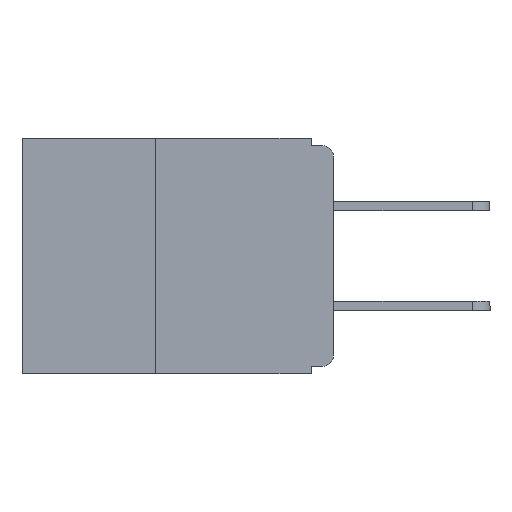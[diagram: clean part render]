
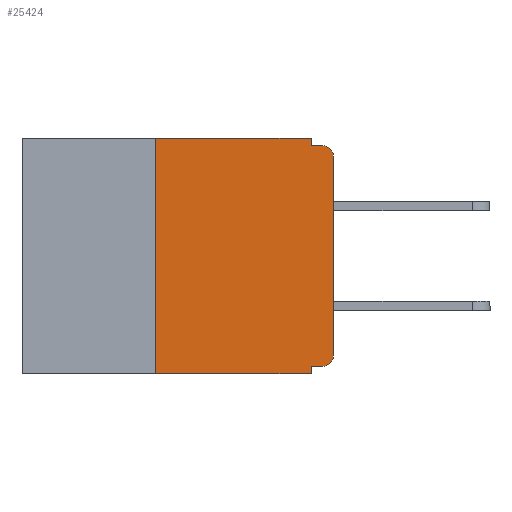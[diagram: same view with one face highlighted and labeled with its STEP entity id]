
A CAD part, left-side view. The second image highlights one B-rep face of the part: STEP entity #25424.
In plain terms, the highlighted planar face has unit normal (-1, 0, 0).
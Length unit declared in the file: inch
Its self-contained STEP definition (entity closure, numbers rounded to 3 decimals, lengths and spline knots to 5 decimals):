
#321 = DIRECTION ( 'NONE',  ( -1., 0., 0. ) ) ;
#1254 = LINE ( 'NONE', #21954, #26834 ) ;
#1456 = VERTEX_POINT ( 'NONE', #5922 ) ;
#1855 = ORIENTED_EDGE ( 'NONE', *, *, #14779, .F. ) ;
#1980 = AXIS2_PLACEMENT_3D ( 'NONE', #15979, #321, #18461 ) ;
#1983 = CARTESIAN_POINT ( 'NONE',  ( 0., 0.031, -0.33 ) ) ;
#2235 = EDGE_CURVE ( 'NONE', #10474, #3486, #18553, .T. ) ;
#2675 = ORIENTED_EDGE ( 'NONE', *, *, #2235, .F. ) ;
#2961 = DIRECTION ( 'NONE',  ( 0., 1., 0. ) ) ;
#3486 = VERTEX_POINT ( 'NONE', #18866 ) ;
#3642 = EDGE_CURVE ( 'NONE', #28663, #19029, #20667, .T. ) ;
#3781 = LINE ( 'NONE', #26192, #21782 ) ;
#4059 = VECTOR ( 'NONE', #2961, 39.37008 ) ;
#4192 = EDGE_CURVE ( 'NONE', #5021, #10474, #3781, .T. ) ;
#4598 = EDGE_LOOP ( 'NONE', ( #18800, #23848, #2675, #14536, #27763, #10139, #29306, #1855, #31661, #23909 ) ) ;
#4897 = PLANE ( 'NONE',  #17253 ) ;
#4975 = VECTOR ( 'NONE', #27396, 39.37008 ) ;
#5006 = CARTESIAN_POINT ( 'NONE',  ( 0., 0.437, -0.33 ) ) ;
#5021 = VERTEX_POINT ( 'NONE', #12494 ) ;
#5922 = CARTESIAN_POINT ( 'NONE',  ( 0., 0.031, -0.33 ) ) ;
#6089 = DIRECTION ( 'NONE',  ( 0., -1., 0. ) ) ;
#6998 = CARTESIAN_POINT ( 'NONE',  ( 0., 0.25, -0.33 ) ) ;
#9578 = EDGE_CURVE ( 'NONE', #31241, #29341, #11056, .T. ) ;
#9633 = DIRECTION ( 'NONE',  ( 0., 0., 1. ) ) ;
#9745 = CIRCLE ( 'NONE', #16161, 0.015 ) ;
#9995 = DIRECTION ( 'NONE',  ( -1., 0., 0. ) ) ;
#10139 = ORIENTED_EDGE ( 'NONE', *, *, #15335, .F. ) ;
#10474 = VERTEX_POINT ( 'NONE', #27161 ) ;
#10807 = CARTESIAN_POINT ( 'NONE',  ( 0., 0., -0.32 ) ) ;
#11056 = LINE ( 'NONE', #10807, #4059 ) ;
#11639 = CARTESIAN_POINT ( 'NONE',  ( 0., 0., -0.025 ) ) ;
#11872 = VERTEX_POINT ( 'NONE', #31697 ) ;
#11895 = DIRECTION ( 'NONE',  ( 0., -1., 0. ) ) ;
#12494 = CARTESIAN_POINT ( 'NONE',  ( 0., 0.031, 0. ) ) ;
#12799 = DIRECTION ( 'NONE',  ( 0., 0., -1. ) ) ;
#13056 = CARTESIAN_POINT ( 'NONE',  ( 0., 0., 0. ) ) ;
#13100 = CARTESIAN_POINT ( 'NONE',  ( 0., 0., -0.01 ) ) ;
#13228 = DIRECTION ( 'NONE',  ( 0., 0., 1. ) ) ;
#13230 = EDGE_CURVE ( 'NONE', #11872, #5021, #1254, .T. ) ;
#13248 = VECTOR ( 'NONE', #13228, 39.37008 ) ;
#14536 = ORIENTED_EDGE ( 'NONE', *, *, #4192, .F. ) ;
#14779 = EDGE_CURVE ( 'NONE', #29341, #1456, #25238, .T. ) ;
#15335 = EDGE_CURVE ( 'NONE', #28297, #11872, #26562, .T. ) ;
#15979 = CARTESIAN_POINT ( 'NONE',  ( 0., 0.015, -0.305 ) ) ;
#16161 = AXIS2_PLACEMENT_3D ( 'NONE', #25021, #9995, #27505 ) ;
#17253 = AXIS2_PLACEMENT_3D ( 'NONE', #30107, #27697, #12799 ) ;
#17553 = CARTESIAN_POINT ( 'NONE',  ( 0., 0., -0.305 ) ) ;
#17620 = LINE ( 'NONE', #5006, #23475 ) ;
#17950 = CARTESIAN_POINT ( 'NONE',  ( 0., 0.25, -0.33 ) ) ;
#18461 = DIRECTION ( 'NONE',  ( 0., 0., -1. ) ) ;
#18553 = LINE ( 'NONE', #13100, #24403 ) ;
#18800 = ORIENTED_EDGE ( 'NONE', *, *, #3642, .T. ) ;
#18866 = CARTESIAN_POINT ( 'NONE',  ( 0., 0.015, -0.01 ) ) ;
#19029 = VERTEX_POINT ( 'NONE', #11639 ) ;
#20667 = LINE ( 'NONE', #13056, #13248 ) ;
#20744 = VECTOR ( 'NONE', #9633, 39.37008 ) ;
#20877 = EDGE_CURVE ( 'NONE', #19029, #3486, #9745, .T. ) ;
#21591 = EDGE_CURVE ( 'NONE', #31241, #28663, #23621, .T. ) ;
#21782 = VECTOR ( 'NONE', #26218, 39.37008 ) ;
#21954 = CARTESIAN_POINT ( 'NONE',  ( 0., 0.437, 0. ) ) ;
#23475 = VECTOR ( 'NONE', #28259, 39.37008 ) ;
#23621 = CIRCLE ( 'NONE', #1980, 0.015 ) ;
#23686 = EDGE_CURVE ( 'NONE', #28297, #1456, #17620, .T. ) ;
#23848 = ORIENTED_EDGE ( 'NONE', *, *, #20877, .T. ) ;
#23909 = ORIENTED_EDGE ( 'NONE', *, *, #21591, .T. ) ;
#24403 = VECTOR ( 'NONE', #6089, 39.37008 ) ;
#25021 = CARTESIAN_POINT ( 'NONE',  ( 0., 0.015, -0.025 ) ) ;
#25238 = LINE ( 'NONE', #1983, #4975 ) ;
#25384 = CARTESIAN_POINT ( 'NONE',  ( 0., 0.031, -0.32 ) ) ;
#25424 = ADVANCED_FACE ( 'NONE', ( #27239 ), #4897, .F. ) ;
#25707 = CARTESIAN_POINT ( 'NONE',  ( 0., 0.015, -0.32 ) ) ;
#26192 = CARTESIAN_POINT ( 'NONE',  ( 0., 0.031, 0. ) ) ;
#26218 = DIRECTION ( 'NONE',  ( 0., 0., -1. ) ) ;
#26562 = LINE ( 'NONE', #6998, #20744 ) ;
#26834 = VECTOR ( 'NONE', #11895, 39.37008 ) ;
#27161 = CARTESIAN_POINT ( 'NONE',  ( 0., 0.031, -0.01 ) ) ;
#27239 = FACE_OUTER_BOUND ( 'NONE', #4598, .T. ) ;
#27396 = DIRECTION ( 'NONE',  ( 0., 0., -1. ) ) ;
#27505 = DIRECTION ( 'NONE',  ( 0., 0., -1. ) ) ;
#27697 = DIRECTION ( 'NONE',  ( 1., 0., 0. ) ) ;
#27763 = ORIENTED_EDGE ( 'NONE', *, *, #13230, .F. ) ;
#28259 = DIRECTION ( 'NONE',  ( 0., -1., 0. ) ) ;
#28297 = VERTEX_POINT ( 'NONE', #17950 ) ;
#28663 = VERTEX_POINT ( 'NONE', #17553 ) ;
#29306 = ORIENTED_EDGE ( 'NONE', *, *, #23686, .T. ) ;
#29341 = VERTEX_POINT ( 'NONE', #25384 ) ;
#30107 = CARTESIAN_POINT ( 'NONE',  ( 0., 0.437, 0. ) ) ;
#31241 = VERTEX_POINT ( 'NONE', #25707 ) ;
#31661 = ORIENTED_EDGE ( 'NONE', *, *, #9578, .F. ) ;
#31697 = CARTESIAN_POINT ( 'NONE',  ( 0., 0.25, 0. ) ) ;
